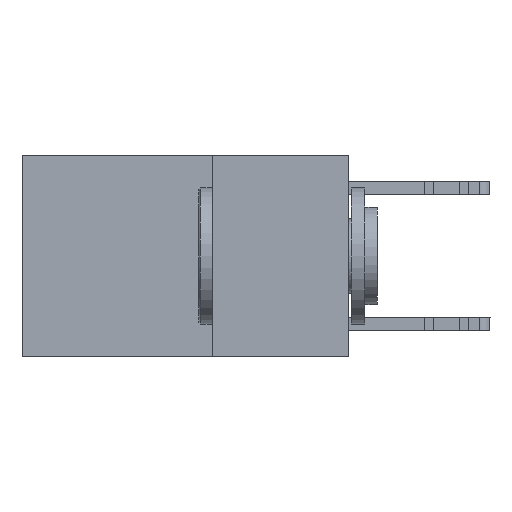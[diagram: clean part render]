
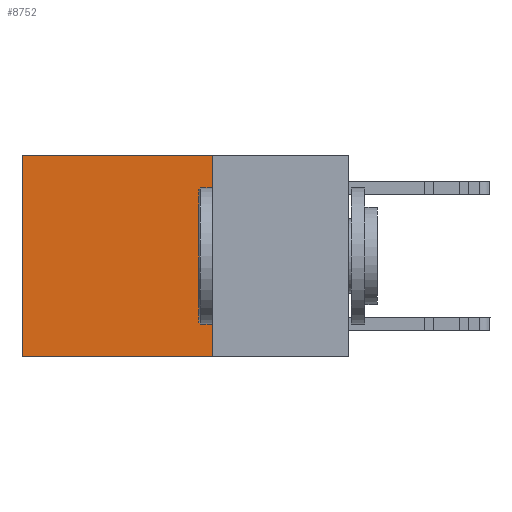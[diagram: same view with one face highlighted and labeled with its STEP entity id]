
A CAD part, left-side view. The second image highlights one B-rep face of the part: STEP entity #8752.
In plain terms, the highlighted planar face has unit normal (-1, 0, 0).
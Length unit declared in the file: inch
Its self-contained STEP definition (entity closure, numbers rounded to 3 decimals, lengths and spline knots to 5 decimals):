
#3903 = EDGE_CURVE ( 'NONE', #27291, #6177, #29615, .T. ) ;
#5140 = ORIENTED_EDGE ( 'NONE', *, *, #6213, .F. ) ;
#5348 = VECTOR ( 'NONE', #24738, 39.37008 ) ;
#6177 = VERTEX_POINT ( 'NONE', #19583 ) ;
#6213 = EDGE_CURVE ( 'NONE', #27291, #16966, #6501, .T. ) ;
#6252 = VECTOR ( 'NONE', #16053, 39.37008 ) ;
#6374 = VECTOR ( 'NONE', #23965, 39.37008 ) ;
#6501 = LINE ( 'NONE', #16265, #6252 ) ;
#7201 = LINE ( 'NONE', #23970, #6374 ) ;
#7623 = CARTESIAN_POINT ( 'NONE',  ( 0.2625, 0.6, 0. ) ) ;
#7704 = ORIENTED_EDGE ( 'NONE', *, *, #10747, .F. ) ;
#8752 = ADVANCED_FACE ( 'NONE', ( #14562 ), #26007, .F. ) ;
#10747 = EDGE_CURVE ( 'NONE', #16966, #25278, #7201, .T. ) ;
#14562 = FACE_OUTER_BOUND ( 'NONE', #15309, .T. ) ;
#15309 = EDGE_LOOP ( 'NONE', ( #29799, #7704, #5140, #15665 ) ) ;
#15665 = ORIENTED_EDGE ( 'NONE', *, *, #3903, .T. ) ;
#16053 = DIRECTION ( 'NONE',  ( 0., 0., -1. ) ) ;
#16265 = CARTESIAN_POINT ( 'NONE',  ( 0.2625, 0.25, 0. ) ) ;
#16508 = DIRECTION ( 'NONE',  ( 0., 1., 0. ) ) ;
#16966 = VERTEX_POINT ( 'NONE', #20040 ) ;
#17113 = CARTESIAN_POINT ( 'NONE',  ( 0.2625, 0.25, 0. ) ) ;
#17287 = CARTESIAN_POINT ( 'NONE',  ( 0.2625, 0.6, -0.37 ) ) ;
#19583 = CARTESIAN_POINT ( 'NONE',  ( 0.2625, 0.6, 0. ) ) ;
#20040 = CARTESIAN_POINT ( 'NONE',  ( 0.2625, 0.25, -0.37 ) ) ;
#22959 = CARTESIAN_POINT ( 'NONE',  ( 0.2625, 0.25, 0. ) ) ;
#23965 = DIRECTION ( 'NONE',  ( 0., 1., 0. ) ) ;
#23970 = CARTESIAN_POINT ( 'NONE',  ( 0.2625, 0.25, -0.37 ) ) ;
#24738 = DIRECTION ( 'NONE',  ( 0., 0., -1. ) ) ;
#25278 = VERTEX_POINT ( 'NONE', #17287 ) ;
#25546 = DIRECTION ( 'NONE',  ( 0., 0., -1. ) ) ;
#25789 = DIRECTION ( 'NONE',  ( 1., 0., 0. ) ) ;
#26007 = PLANE ( 'NONE',  #26993 ) ;
#26722 = CARTESIAN_POINT ( 'NONE',  ( 0.2625, 0.25, 0. ) ) ;
#26993 = AXIS2_PLACEMENT_3D ( 'NONE', #26722, #25789, #25546 ) ;
#27291 = VERTEX_POINT ( 'NONE', #22959 ) ;
#29539 = VECTOR ( 'NONE', #16508, 39.37008 ) ;
#29615 = LINE ( 'NONE', #17113, #29539 ) ;
#29752 = LINE ( 'NONE', #7623, #5348 ) ;
#29799 = ORIENTED_EDGE ( 'NONE', *, *, #30707, .T. ) ;
#30707 = EDGE_CURVE ( 'NONE', #6177, #25278, #29752, .T. ) ;
